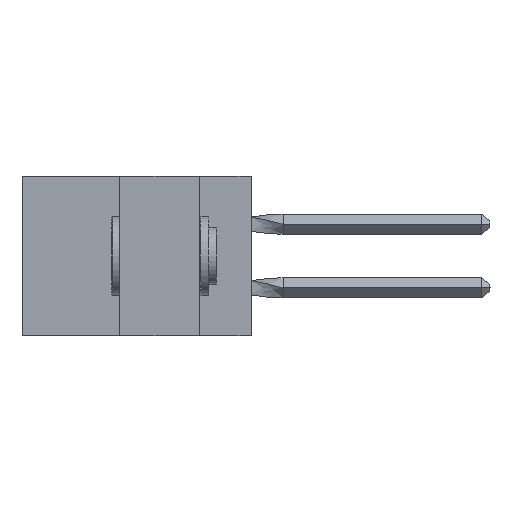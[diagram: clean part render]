
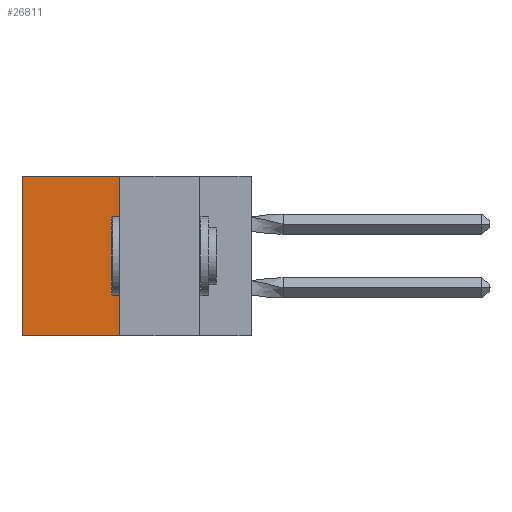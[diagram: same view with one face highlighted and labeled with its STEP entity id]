
A CAD part, left-side view. The second image highlights one B-rep face of the part: STEP entity #26811.
In plain terms, the highlighted planar face has unit normal (-1, 0, 0).
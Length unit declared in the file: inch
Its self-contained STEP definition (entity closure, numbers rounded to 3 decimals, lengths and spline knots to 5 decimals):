
#1388 = LINE ( 'NONE', #8208, #9605 ) ;
#1430 = VERTEX_POINT ( 'NONE', #22686 ) ;
#1686 = LINE ( 'NONE', #8585, #22877 ) ;
#2747 = DIRECTION ( 'NONE',  ( 1., 0., 0. ) ) ;
#4802 = CARTESIAN_POINT ( 'NONE',  ( 0.305, 0.413, -0.5 ) ) ;
#5098 = CARTESIAN_POINT ( 'NONE',  ( 0.305, 0.413, 0. ) ) ;
#5554 = CARTESIAN_POINT ( 'NONE',  ( 0.305, 0.413, -0.5 ) ) ;
#6191 = AXIS2_PLACEMENT_3D ( 'NONE', #4802, #2747, #12566 ) ;
#6243 = DIRECTION ( 'NONE',  ( 0., 1., 0. ) ) ;
#6894 = VERTEX_POINT ( 'NONE', #14232 ) ;
#7687 = LINE ( 'NONE', #5554, #17105 ) ;
#8208 = CARTESIAN_POINT ( 'NONE',  ( 0.305, 0.72, -0.5 ) ) ;
#8585 = CARTESIAN_POINT ( 'NONE',  ( 0.305, 0.413, -0.5 ) ) ;
#9605 = VECTOR ( 'NONE', #15551, 39.37008 ) ;
#10710 = EDGE_CURVE ( 'NONE', #11605, #6894, #7687, .T. ) ;
#11605 = VERTEX_POINT ( 'NONE', #18021 ) ;
#12566 = DIRECTION ( 'NONE',  ( 0., 0., -1. ) ) ;
#13054 = DIRECTION ( 'NONE',  ( 0., 1., 0. ) ) ;
#14232 = CARTESIAN_POINT ( 'NONE',  ( 0.305, 0.413, -0.5 ) ) ;
#15551 = DIRECTION ( 'NONE',  ( 0., 0., -1. ) ) ;
#16260 = ORIENTED_EDGE ( 'NONE', *, *, #22277, .T. ) ;
#16592 = ORIENTED_EDGE ( 'NONE', *, *, #18059, .T. ) ;
#17105 = VECTOR ( 'NONE', #17359, 39.37008 ) ;
#17168 = EDGE_LOOP ( 'NONE', ( #16260, #30050, #22223, #16592 ) ) ;
#17359 = DIRECTION ( 'NONE',  ( 0., 0., -1. ) ) ;
#18021 = CARTESIAN_POINT ( 'NONE',  ( 0.305, 0.413, 0. ) ) ;
#18059 = EDGE_CURVE ( 'NONE', #11605, #30303, #26298, .T. ) ;
#19867 = EDGE_CURVE ( 'NONE', #6894, #1430, #1686, .T. ) ;
#22223 = ORIENTED_EDGE ( 'NONE', *, *, #10710, .F. ) ;
#22277 = EDGE_CURVE ( 'NONE', #30303, #1430, #1388, .T. ) ;
#22686 = CARTESIAN_POINT ( 'NONE',  ( 0.305, 0.72, -0.5 ) ) ;
#22877 = VECTOR ( 'NONE', #6243, 39.37008 ) ;
#24471 = VECTOR ( 'NONE', #13054, 39.37008 ) ;
#26298 = LINE ( 'NONE', #5098, #24471 ) ;
#26662 = PLANE ( 'NONE',  #6191 ) ;
#26811 = ADVANCED_FACE ( 'NONE', ( #28245 ), #26662, .F. ) ;
#28245 = FACE_OUTER_BOUND ( 'NONE', #17168, .T. ) ;
#30050 = ORIENTED_EDGE ( 'NONE', *, *, #19867, .F. ) ;
#30303 = VERTEX_POINT ( 'NONE', #31229 ) ;
#31229 = CARTESIAN_POINT ( 'NONE',  ( 0.305, 0.72, 0. ) ) ;
